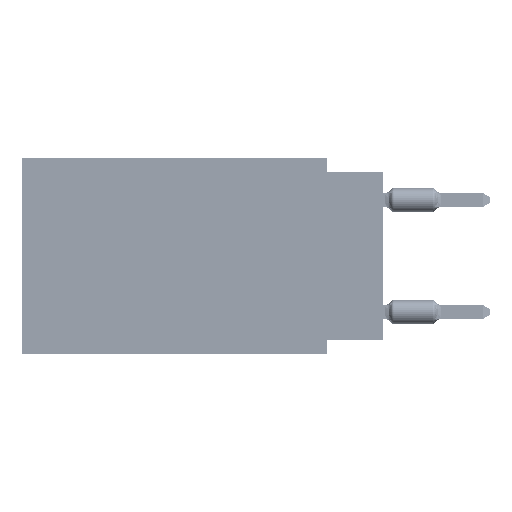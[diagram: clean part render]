
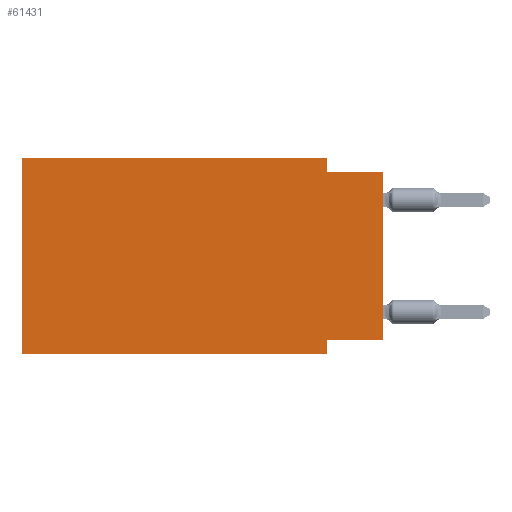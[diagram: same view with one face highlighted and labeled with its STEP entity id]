
A CAD part, left-side view. The second image highlights one B-rep face of the part: STEP entity #61431.
In plain terms, the highlighted planar face has unit normal (-1, 0, 0).
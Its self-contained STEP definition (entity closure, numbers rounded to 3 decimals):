
#641 = CARTESIAN_POINT ( 'NONE',  ( 0., 2.54, -8.89 ) ) ;
#967 = DIRECTION ( 'NONE',  ( 0., -1., 0. ) ) ;
#2855 = VERTEX_POINT ( 'NONE', #50907 ) ;
#3635 = CARTESIAN_POINT ( 'NONE',  ( 0., 16.383, 0. ) ) ;
#4850 = DIRECTION ( 'NONE',  ( 0., 1., 0. ) ) ;
#5006 = DIRECTION ( 'NONE',  ( 0., 0., 1. ) ) ;
#5951 = DIRECTION ( 'NONE',  ( 0., 0., -1. ) ) ;
#6465 = CARTESIAN_POINT ( 'NONE',  ( 0., 0., 0. ) ) ;
#7048 = ORIENTED_EDGE ( 'NONE', *, *, #42282, .F. ) ;
#8408 = VECTOR ( 'NONE', #52490, 1000. ) ;
#8513 = ORIENTED_EDGE ( 'NONE', *, *, #18870, .F. ) ;
#9262 = EDGE_CURVE ( 'NONE', #2855, #34372, #20642, .T. ) ;
#10411 = EDGE_CURVE ( 'NONE', #43842, #34372, #32827, .T. ) ;
#10659 = CARTESIAN_POINT ( 'NONE',  ( 0., 0., -0.635 ) ) ;
#11165 = LINE ( 'NONE', #6465, #32262 ) ;
#11591 = CARTESIAN_POINT ( 'NONE',  ( 0., 0., -8.255 ) ) ;
#14275 = CARTESIAN_POINT ( 'NONE',  ( 0., 16.383, 0. ) ) ;
#14788 = LINE ( 'NONE', #33827, #16710 ) ;
#15667 = EDGE_CURVE ( 'NONE', #40005, #34680, #14788, .T. ) ;
#16710 = VECTOR ( 'NONE', #52867, 1000. ) ;
#18050 = CARTESIAN_POINT ( 'NONE',  ( 0., 2.54, -0.635 ) ) ;
#18656 = PLANE ( 'NONE',  #21016 ) ;
#18870 = EDGE_CURVE ( 'NONE', #26664, #40005, #22330, .T. ) ;
#20642 = LINE ( 'NONE', #641, #28204 ) ;
#21016 = AXIS2_PLACEMENT_3D ( 'NONE', #14275, #32395, #23026 ) ;
#22303 = ORIENTED_EDGE ( 'NONE', *, *, #15667, .F. ) ;
#22330 = LINE ( 'NONE', #60435, #56848 ) ;
#23026 = DIRECTION ( 'NONE',  ( 0., 0., -1. ) ) ;
#25518 = DIRECTION ( 'NONE',  ( 0., 0., 1. ) ) ;
#25652 = ORIENTED_EDGE ( 'NONE', *, *, #9262, .F. ) ;
#25922 = CARTESIAN_POINT ( 'NONE',  ( 0., 0., -0.635 ) ) ;
#26664 = VERTEX_POINT ( 'NONE', #3635 ) ;
#27520 = EDGE_CURVE ( 'NONE', #34680, #49734, #57497, .T. ) ;
#28204 = VECTOR ( 'NONE', #5951, 1000. ) ;
#28729 = CARTESIAN_POINT ( 'NONE',  ( 0., 2.54, -8.89 ) ) ;
#29065 = LINE ( 'NONE', #38420, #54242 ) ;
#29509 = ORIENTED_EDGE ( 'NONE', *, *, #34213, .T. ) ;
#30325 = VECTOR ( 'NONE', #4850, 1000. ) ;
#32262 = VECTOR ( 'NONE', #25518, 1000. ) ;
#32395 = DIRECTION ( 'NONE',  ( 1., 0., 0. ) ) ;
#32793 = ORIENTED_EDGE ( 'NONE', *, *, #41897, .F. ) ;
#32827 = LINE ( 'NONE', #57501, #8408 ) ;
#33827 = CARTESIAN_POINT ( 'NONE',  ( 0., 2.54, 0. ) ) ;
#34213 = EDGE_CURVE ( 'NONE', #60871, #49734, #11165, .T. ) ;
#34372 = VERTEX_POINT ( 'NONE', #28729 ) ;
#34680 = VERTEX_POINT ( 'NONE', #18050 ) ;
#36159 = CARTESIAN_POINT ( 'NONE',  ( 0., 16.383, -8.89 ) ) ;
#38420 = CARTESIAN_POINT ( 'NONE',  ( 0., 16.383, 0. ) ) ;
#38543 = ORIENTED_EDGE ( 'NONE', *, *, #10411, .T. ) ;
#40005 = VERTEX_POINT ( 'NONE', #53626 ) ;
#40681 = VECTOR ( 'NONE', #967, 1000. ) ;
#41897 = EDGE_CURVE ( 'NONE', #60871, #2855, #52315, .T. ) ;
#42282 = EDGE_CURVE ( 'NONE', #43842, #26664, #29065, .T. ) ;
#43459 = EDGE_LOOP ( 'NONE', ( #29509, #54775, #22303, #8513, #7048, #38543, #25652, #32793 ) ) ;
#43842 = VERTEX_POINT ( 'NONE', #36159 ) ;
#47620 = CARTESIAN_POINT ( 'NONE',  ( 0., 0., -8.255 ) ) ;
#49734 = VERTEX_POINT ( 'NONE', #25922 ) ;
#50907 = CARTESIAN_POINT ( 'NONE',  ( 0., 2.54, -8.255 ) ) ;
#52315 = LINE ( 'NONE', #47620, #30325 ) ;
#52490 = DIRECTION ( 'NONE',  ( 0., -1., 0. ) ) ;
#52867 = DIRECTION ( 'NONE',  ( 0., 0., -1. ) ) ;
#53626 = CARTESIAN_POINT ( 'NONE',  ( 0., 2.54, 0. ) ) ;
#54242 = VECTOR ( 'NONE', #5006, 1000. ) ;
#54775 = ORIENTED_EDGE ( 'NONE', *, *, #27520, .F. ) ;
#56848 = VECTOR ( 'NONE', #59510, 1000. ) ;
#57049 = FACE_OUTER_BOUND ( 'NONE', #43459, .T. ) ;
#57497 = LINE ( 'NONE', #10659, #40681 ) ;
#57501 = CARTESIAN_POINT ( 'NONE',  ( 0., 16.383, -8.89 ) ) ;
#59510 = DIRECTION ( 'NONE',  ( 0., -1., 0. ) ) ;
#60435 = CARTESIAN_POINT ( 'NONE',  ( 0., 16.383, 0. ) ) ;
#60871 = VERTEX_POINT ( 'NONE', #11591 ) ;
#61431 = ADVANCED_FACE ( 'NONE', ( #57049 ), #18656, .F. ) ;
